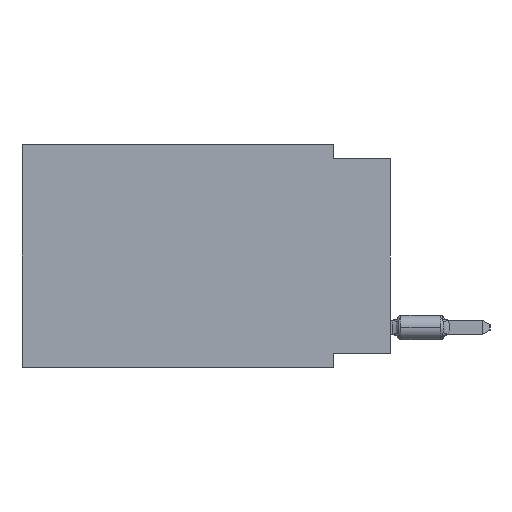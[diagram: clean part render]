
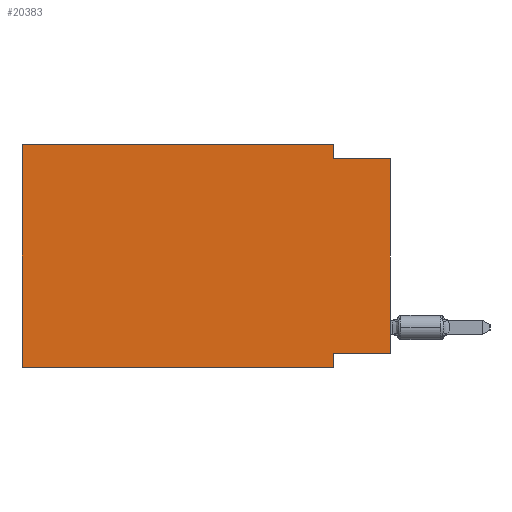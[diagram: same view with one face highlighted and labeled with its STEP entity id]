
A CAD part, left-side view. The second image highlights one B-rep face of the part: STEP entity #20383.
In plain terms, the highlighted planar face has unit normal (-1, 0, 0).
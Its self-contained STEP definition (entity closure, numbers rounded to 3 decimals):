
#41 = CARTESIAN_POINT ( 'NONE',  ( 0., 2.54, 0. ) ) ;
#304 = DIRECTION ( 'NONE',  ( 0., 0., -1. ) ) ;
#338 = CARTESIAN_POINT ( 'NONE',  ( 0., 2.54, -9.906 ) ) ;
#397 = EDGE_CURVE ( 'NONE', #16884, #24174, #14772, .T. ) ;
#588 = EDGE_CURVE ( 'NONE', #2116, #24174, #16711, .T. ) ;
#2116 = VERTEX_POINT ( 'NONE', #18109 ) ;
#2126 = VECTOR ( 'NONE', #304, 1000. ) ;
#2399 = EDGE_CURVE ( 'NONE', #16627, #2116, #20900, .T. ) ;
#2890 = VECTOR ( 'NONE', #33054, 1000. ) ;
#2996 = CARTESIAN_POINT ( 'NONE',  ( 0., 16.383, 0. ) ) ;
#5446 = CARTESIAN_POINT ( 'NONE',  ( 0., 2.54, 0. ) ) ;
#6636 = LINE ( 'NONE', #19041, #12001 ) ;
#6954 = DIRECTION ( 'NONE',  ( 0., 0., -1. ) ) ;
#7433 = EDGE_LOOP ( 'NONE', ( #19013, #18155, #19488, #34133, #31792, #16269, #26292, #24539 ) ) ;
#7561 = VECTOR ( 'NONE', #11400, 1000. ) ;
#8468 = VERTEX_POINT ( 'NONE', #41 ) ;
#11333 = DIRECTION ( 'NONE',  ( 0., -1., 0. ) ) ;
#11400 = DIRECTION ( 'NONE',  ( 0., 1., 0. ) ) ;
#11439 = CARTESIAN_POINT ( 'NONE',  ( 0., 16.383, 0. ) ) ;
#11701 = EDGE_CURVE ( 'NONE', #16884, #19228, #14682, .T. ) ;
#11936 = CARTESIAN_POINT ( 'NONE',  ( 0., 16.383, 0. ) ) ;
#12001 = VECTOR ( 'NONE', #25314, 1000. ) ;
#12781 = CARTESIAN_POINT ( 'NONE',  ( 0., 16.383, 0. ) ) ;
#14682 = LINE ( 'NONE', #11439, #30195 ) ;
#14772 = LINE ( 'NONE', #39138, #37929 ) ;
#16269 = ORIENTED_EDGE ( 'NONE', *, *, #397, .T. ) ;
#16627 = VERTEX_POINT ( 'NONE', #21149 ) ;
#16661 = CARTESIAN_POINT ( 'NONE',  ( 0., 16.383, -9.906 ) ) ;
#16711 = LINE ( 'NONE', #22997, #25628 ) ;
#16884 = VERTEX_POINT ( 'NONE', #16661 ) ;
#18109 = CARTESIAN_POINT ( 'NONE',  ( 0., 2.54, -9.271 ) ) ;
#18155 = ORIENTED_EDGE ( 'NONE', *, *, #39948, .F. ) ;
#19013 = ORIENTED_EDGE ( 'NONE', *, *, #39709, .T. ) ;
#19041 = CARTESIAN_POINT ( 'NONE',  ( 0., 0., -0.635 ) ) ;
#19228 = VERTEX_POINT ( 'NONE', #12781 ) ;
#19488 = ORIENTED_EDGE ( 'NONE', *, *, #35914, .F. ) ;
#20383 = ADVANCED_FACE ( 'NONE', ( #33464 ), #27359, .F. ) ;
#20766 = DIRECTION ( 'NONE',  ( 0., 0., 1. ) ) ;
#20900 = LINE ( 'NONE', #33297, #7561 ) ;
#21028 = CARTESIAN_POINT ( 'NONE',  ( 0., 0., -0.635 ) ) ;
#21149 = CARTESIAN_POINT ( 'NONE',  ( 0., 0., -9.271 ) ) ;
#21478 = LINE ( 'NONE', #2996, #37256 ) ;
#22997 = CARTESIAN_POINT ( 'NONE',  ( 0., 2.54, -9.906 ) ) ;
#23722 = CARTESIAN_POINT ( 'NONE',  ( 0., 0., 0. ) ) ;
#24174 = VERTEX_POINT ( 'NONE', #338 ) ;
#24322 = DIRECTION ( 'NONE',  ( 0., 0., -1. ) ) ;
#24539 = ORIENTED_EDGE ( 'NONE', *, *, #2399, .F. ) ;
#24883 = AXIS2_PLACEMENT_3D ( 'NONE', #11936, #33044, #24322 ) ;
#25314 = DIRECTION ( 'NONE',  ( 0., -1., 0. ) ) ;
#25628 = VECTOR ( 'NONE', #6954, 1000. ) ;
#25638 = VERTEX_POINT ( 'NONE', #38288 ) ;
#26292 = ORIENTED_EDGE ( 'NONE', *, *, #588, .F. ) ;
#27359 = PLANE ( 'NONE',  #24883 ) ;
#27779 = DIRECTION ( 'NONE',  ( 0., -1., 0. ) ) ;
#28148 = LINE ( 'NONE', #5446, #2126 ) ;
#30195 = VECTOR ( 'NONE', #20766, 1000. ) ;
#31792 = ORIENTED_EDGE ( 'NONE', *, *, #11701, .F. ) ;
#33044 = DIRECTION ( 'NONE',  ( 1., 0., 0. ) ) ;
#33054 = DIRECTION ( 'NONE',  ( 0., 0., 1. ) ) ;
#33297 = CARTESIAN_POINT ( 'NONE',  ( 0., 0., -9.271 ) ) ;
#33431 = VERTEX_POINT ( 'NONE', #21028 ) ;
#33464 = FACE_OUTER_BOUND ( 'NONE', #7433, .T. ) ;
#34133 = ORIENTED_EDGE ( 'NONE', *, *, #34399, .F. ) ;
#34399 = EDGE_CURVE ( 'NONE', #19228, #8468, #21478, .T. ) ;
#35914 = EDGE_CURVE ( 'NONE', #8468, #25638, #28148, .T. ) ;
#37256 = VECTOR ( 'NONE', #27779, 1000. ) ;
#37929 = VECTOR ( 'NONE', #11333, 1000. ) ;
#38288 = CARTESIAN_POINT ( 'NONE',  ( 0., 2.54, -0.635 ) ) ;
#39138 = CARTESIAN_POINT ( 'NONE',  ( 0., 16.383, -9.906 ) ) ;
#39142 = LINE ( 'NONE', #23722, #2890 ) ;
#39709 = EDGE_CURVE ( 'NONE', #16627, #33431, #39142, .T. ) ;
#39948 = EDGE_CURVE ( 'NONE', #25638, #33431, #6636, .T. ) ;
